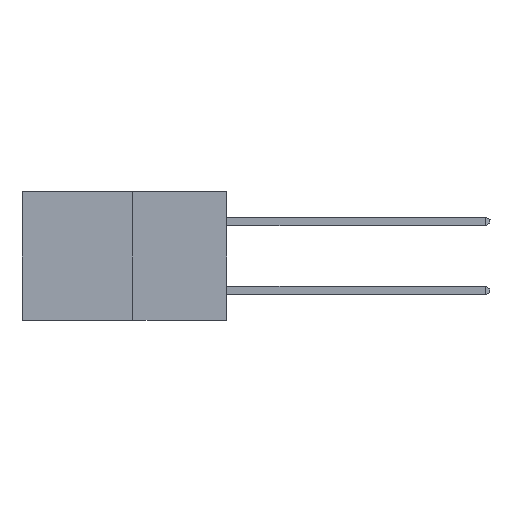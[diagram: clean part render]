
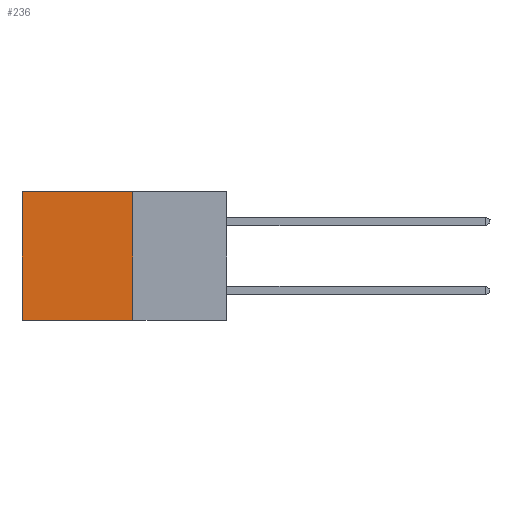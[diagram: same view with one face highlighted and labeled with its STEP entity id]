
A CAD part, left-side view. The second image highlights one B-rep face of the part: STEP entity #236.
In plain terms, the highlighted planar face has unit normal (-1, 0, 0).
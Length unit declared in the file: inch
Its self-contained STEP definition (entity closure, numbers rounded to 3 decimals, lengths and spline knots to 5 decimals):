
#227 = DIRECTION ( 'NONE',  ( 0., 0., -1. ) ) ;
#236 = ADVANCED_FACE ( 'NONE', ( #14344 ), #4678, .F. ) ;
#839 = VERTEX_POINT ( 'NONE', #6298 ) ;
#2113 = EDGE_LOOP ( 'NONE', ( #18104, #21150, #13605, #19964 ) ) ;
#2510 = DIRECTION ( 'NONE',  ( 0., 0., -1. ) ) ;
#2545 = LINE ( 'NONE', #17128, #12261 ) ;
#3644 = DIRECTION ( 'NONE',  ( 0., 1., 0. ) ) ;
#4201 = EDGE_CURVE ( 'NONE', #6766, #839, #7834, .T. ) ;
#4678 = PLANE ( 'NONE',  #11045 ) ;
#5782 = VECTOR ( 'NONE', #24652, 39.37008 ) ;
#6298 = CARTESIAN_POINT ( 'NONE',  ( 0.277, 0.27, -0.37 ) ) ;
#6730 = CARTESIAN_POINT ( 'NONE',  ( 0.277, 0.27, 0. ) ) ;
#6766 = VERTEX_POINT ( 'NONE', #10645 ) ;
#7217 = VECTOR ( 'NONE', #2510, 39.37008 ) ;
#7834 = LINE ( 'NONE', #22838, #7217 ) ;
#8700 = DIRECTION ( 'NONE',  ( 0., 1., 0. ) ) ;
#9556 = CARTESIAN_POINT ( 'NONE',  ( 0.277, 0.59, -0.37 ) ) ;
#9949 = VECTOR ( 'NONE', #8700, 39.37008 ) ;
#10645 = CARTESIAN_POINT ( 'NONE',  ( 0.277, 0.27, 0. ) ) ;
#11045 = AXIS2_PLACEMENT_3D ( 'NONE', #18204, #15177, #227 ) ;
#11569 = LINE ( 'NONE', #9556, #5782 ) ;
#11986 = EDGE_CURVE ( 'NONE', #839, #20239, #2545, .T. ) ;
#12261 = VECTOR ( 'NONE', #3644, 39.37008 ) ;
#13605 = ORIENTED_EDGE ( 'NONE', *, *, #4201, .F. ) ;
#14344 = FACE_OUTER_BOUND ( 'NONE', #2113, .T. ) ;
#14377 = VERTEX_POINT ( 'NONE', #19678 ) ;
#15177 = DIRECTION ( 'NONE',  ( 1., 0., 0. ) ) ;
#16548 = EDGE_CURVE ( 'NONE', #6766, #14377, #20038, .T. ) ;
#17128 = CARTESIAN_POINT ( 'NONE',  ( 0.277, 0.27, -0.37 ) ) ;
#18104 = ORIENTED_EDGE ( 'NONE', *, *, #22346, .T. ) ;
#18204 = CARTESIAN_POINT ( 'NONE',  ( 0.277, 0.27, -0.37 ) ) ;
#19678 = CARTESIAN_POINT ( 'NONE',  ( 0.277, 0.59, 0. ) ) ;
#19964 = ORIENTED_EDGE ( 'NONE', *, *, #16548, .T. ) ;
#20038 = LINE ( 'NONE', #6730, #9949 ) ;
#20239 = VERTEX_POINT ( 'NONE', #22223 ) ;
#21150 = ORIENTED_EDGE ( 'NONE', *, *, #11986, .F. ) ;
#22223 = CARTESIAN_POINT ( 'NONE',  ( 0.277, 0.59, -0.37 ) ) ;
#22346 = EDGE_CURVE ( 'NONE', #14377, #20239, #11569, .T. ) ;
#22838 = CARTESIAN_POINT ( 'NONE',  ( 0.277, 0.27, -0.37 ) ) ;
#24652 = DIRECTION ( 'NONE',  ( 0., 0., -1. ) ) ;
